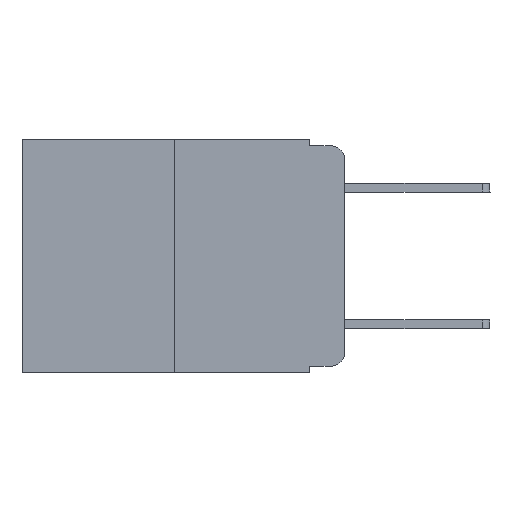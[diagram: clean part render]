
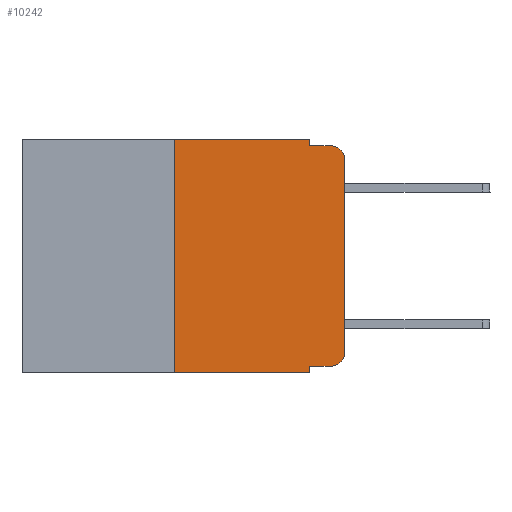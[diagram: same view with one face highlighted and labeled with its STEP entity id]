
A CAD part, left-side view. The second image highlights one B-rep face of the part: STEP entity #10242.
In plain terms, the highlighted planar face has unit normal (-1, 0, 0).
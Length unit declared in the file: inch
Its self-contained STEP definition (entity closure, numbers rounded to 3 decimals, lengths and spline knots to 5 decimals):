
#24 = CARTESIAN_POINT ( 'NONE',  ( 0., 0.051, -0.01 ) ) ;
#63 = LINE ( 'NONE', #3667, #1178 ) ;
#92 = CARTESIAN_POINT ( 'NONE',  ( 0., 0.473, 0. ) ) ;
#105 = VECTOR ( 'NONE', #903, 39.37008 ) ;
#124 = CARTESIAN_POINT ( 'NONE',  ( 0., 0.25, -0.343 ) ) ;
#150 = FACE_OUTER_BOUND ( 'NONE', #9385, .T. ) ;
#331 = EDGE_CURVE ( 'NONE', #11292, #2616, #63, .T. ) ;
#465 = CARTESIAN_POINT ( 'NONE',  ( 0., 0.051, -0.01 ) ) ;
#477 = DIRECTION ( 'NONE',  ( 0., -1., 0. ) ) ;
#903 = DIRECTION ( 'NONE',  ( 0., -1., 0. ) ) ;
#907 = ORIENTED_EDGE ( 'NONE', *, *, #3565, .F. ) ;
#1026 = VERTEX_POINT ( 'NONE', #5296 ) ;
#1110 = EDGE_CURVE ( 'NONE', #10248, #5178, #7412, .T. ) ;
#1178 = VECTOR ( 'NONE', #6407, 39.37008 ) ;
#1247 = VECTOR ( 'NONE', #477, 39.37008 ) ;
#1381 = CARTESIAN_POINT ( 'NONE',  ( 0., 0.473, 0. ) ) ;
#1452 = DIRECTION ( 'NONE',  ( -1., 0., 0. ) ) ;
#1596 = ORIENTED_EDGE ( 'NONE', *, *, #8710, .T. ) ;
#1679 = VECTOR ( 'NONE', #5575, 39.37008 ) ;
#1703 = AXIS2_PLACEMENT_3D ( 'NONE', #6845, #1452, #4004 ) ;
#1735 = ORIENTED_EDGE ( 'NONE', *, *, #7747, .F. ) ;
#1781 = LINE ( 'NONE', #7111, #9793 ) ;
#1789 = LINE ( 'NONE', #24, #105 ) ;
#2225 = CARTESIAN_POINT ( 'NONE',  ( 0., 0.051, 0. ) ) ;
#2418 = DIRECTION ( 'NONE',  ( 0., -1., 0. ) ) ;
#2450 = CIRCLE ( 'NONE', #1703, 0.02 ) ;
#2535 = CARTESIAN_POINT ( 'NONE',  ( 0., 0.051, -0.333 ) ) ;
#2605 = DIRECTION ( 'NONE',  ( 0., 0., 1. ) ) ;
#2614 = DIRECTION ( 'NONE',  ( 0., 0., -1. ) ) ;
#2616 = VERTEX_POINT ( 'NONE', #7429 ) ;
#2700 = CARTESIAN_POINT ( 'NONE',  ( 0., 0.051, -0.333 ) ) ;
#2975 = ORIENTED_EDGE ( 'NONE', *, *, #6238, .T. ) ;
#3176 = VECTOR ( 'NONE', #8864, 39.37008 ) ;
#3529 = CARTESIAN_POINT ( 'NONE',  ( 0., 0., -0.313 ) ) ;
#3565 = EDGE_CURVE ( 'NONE', #9151, #10248, #7775, .T. ) ;
#3667 = CARTESIAN_POINT ( 'NONE',  ( 0., 0., 0. ) ) ;
#3690 = CARTESIAN_POINT ( 'NONE',  ( 0., 0.02, -0.03 ) ) ;
#3728 = VERTEX_POINT ( 'NONE', #124 ) ;
#3938 = PLANE ( 'NONE',  #11159 ) ;
#4004 = DIRECTION ( 'NONE',  ( 0., 0., -1. ) ) ;
#4920 = EDGE_CURVE ( 'NONE', #5178, #9214, #1789, .T. ) ;
#5178 = VERTEX_POINT ( 'NONE', #465 ) ;
#5281 = CARTESIAN_POINT ( 'NONE',  ( 0., 0.02, -0.01 ) ) ;
#5296 = CARTESIAN_POINT ( 'NONE',  ( 0., 0.02, -0.333 ) ) ;
#5527 = DIRECTION ( 'NONE',  ( -1., 0., 0. ) ) ;
#5575 = DIRECTION ( 'NONE',  ( 0., 0., -1. ) ) ;
#6238 = EDGE_CURVE ( 'NONE', #2616, #9214, #8895, .T. ) ;
#6407 = DIRECTION ( 'NONE',  ( 0., 0., 1. ) ) ;
#6418 = VECTOR ( 'NONE', #2605, 39.37008 ) ;
#6452 = VECTOR ( 'NONE', #2418, 39.37008 ) ;
#6769 = ORIENTED_EDGE ( 'NONE', *, *, #6933, .T. ) ;
#6845 = CARTESIAN_POINT ( 'NONE',  ( 0., 0.02, -0.313 ) ) ;
#6933 = EDGE_CURVE ( 'NONE', #3728, #10118, #10538, .T. ) ;
#7024 = VERTEX_POINT ( 'NONE', #2535 ) ;
#7046 = ORIENTED_EDGE ( 'NONE', *, *, #331, .T. ) ;
#7111 = CARTESIAN_POINT ( 'NONE',  ( 0., 0.051, 0. ) ) ;
#7203 = LINE ( 'NONE', #2700, #3176 ) ;
#7348 = ORIENTED_EDGE ( 'NONE', *, *, #1110, .F. ) ;
#7412 = LINE ( 'NONE', #10090, #1679 ) ;
#7429 = CARTESIAN_POINT ( 'NONE',  ( 0., 0., -0.03 ) ) ;
#7552 = AXIS2_PLACEMENT_3D ( 'NONE', #3690, #5527, #10097 ) ;
#7747 = EDGE_CURVE ( 'NONE', #7024, #10118, #1781, .T. ) ;
#7775 = LINE ( 'NONE', #1381, #1247 ) ;
#8050 = LINE ( 'NONE', #8168, #6418 ) ;
#8168 = CARTESIAN_POINT ( 'NONE',  ( 0., 0.25, 0. ) ) ;
#8190 = ORIENTED_EDGE ( 'NONE', *, *, #9537, .F. ) ;
#8561 = DIRECTION ( 'NONE',  ( 0., 0., -1. ) ) ;
#8710 = EDGE_CURVE ( 'NONE', #7024, #1026, #7203, .T. ) ;
#8864 = DIRECTION ( 'NONE',  ( 0., -1., 0. ) ) ;
#8895 = CIRCLE ( 'NONE', #7552, 0.02 ) ;
#9147 = DIRECTION ( 'NONE',  ( 1., 0., 0. ) ) ;
#9151 = VERTEX_POINT ( 'NONE', #10802 ) ;
#9214 = VERTEX_POINT ( 'NONE', #5281 ) ;
#9385 = EDGE_LOOP ( 'NONE', ( #7046, #2975, #10759, #7348, #907, #8190, #6769, #1735, #1596, #11004 ) ) ;
#9537 = EDGE_CURVE ( 'NONE', #3728, #9151, #8050, .T. ) ;
#9793 = VECTOR ( 'NONE', #2614, 39.37008 ) ;
#10090 = CARTESIAN_POINT ( 'NONE',  ( 0., 0.051, 0. ) ) ;
#10097 = DIRECTION ( 'NONE',  ( 0., 0., -1. ) ) ;
#10118 = VERTEX_POINT ( 'NONE', #11054 ) ;
#10242 = ADVANCED_FACE ( 'NONE', ( #150 ), #3938, .F. ) ;
#10248 = VERTEX_POINT ( 'NONE', #2225 ) ;
#10296 = EDGE_CURVE ( 'NONE', #1026, #11292, #2450, .T. ) ;
#10538 = LINE ( 'NONE', #11430, #6452 ) ;
#10759 = ORIENTED_EDGE ( 'NONE', *, *, #4920, .F. ) ;
#10802 = CARTESIAN_POINT ( 'NONE',  ( 0., 0.25, 0. ) ) ;
#11004 = ORIENTED_EDGE ( 'NONE', *, *, #10296, .T. ) ;
#11054 = CARTESIAN_POINT ( 'NONE',  ( 0., 0.051, -0.343 ) ) ;
#11159 = AXIS2_PLACEMENT_3D ( 'NONE', #92, #9147, #8561 ) ;
#11292 = VERTEX_POINT ( 'NONE', #3529 ) ;
#11430 = CARTESIAN_POINT ( 'NONE',  ( 0., 0.473, -0.343 ) ) ;
